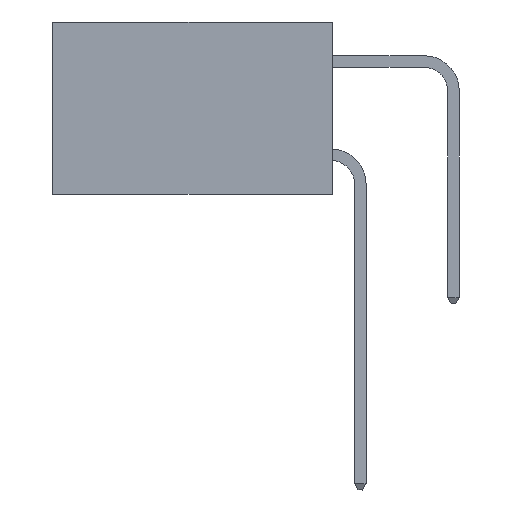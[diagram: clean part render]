
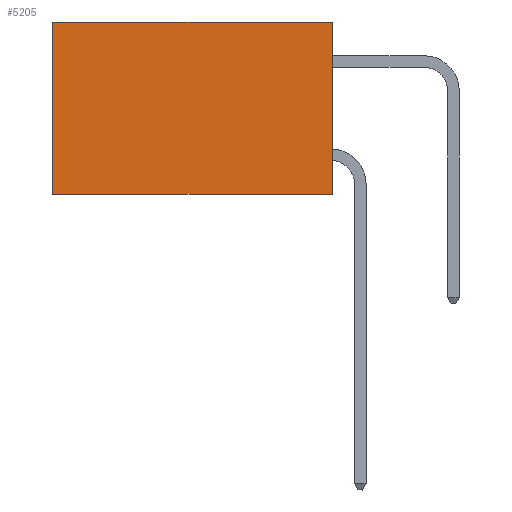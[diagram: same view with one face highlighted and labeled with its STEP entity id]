
A CAD part, left-side view. The second image highlights one B-rep face of the part: STEP entity #5205.
In plain terms, the highlighted planar face has unit normal (-1, 0, 0).
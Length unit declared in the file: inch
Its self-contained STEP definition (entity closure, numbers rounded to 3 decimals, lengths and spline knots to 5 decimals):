
#835 = LINE ( 'NONE', #24938, #24737 ) ;
#1611 = ORIENTED_EDGE ( 'NONE', *, *, #6503, .T. ) ;
#2766 = CARTESIAN_POINT ( 'NONE',  ( 0.298, 0., 0. ) ) ;
#2783 = LINE ( 'NONE', #4137, #17684 ) ;
#2809 = VERTEX_POINT ( 'NONE', #4584 ) ;
#3131 = VERTEX_POINT ( 'NONE', #24430 ) ;
#3649 = ORIENTED_EDGE ( 'NONE', *, *, #23106, .F. ) ;
#3903 = VECTOR ( 'NONE', #14174, 39.37008 ) ;
#4137 = CARTESIAN_POINT ( 'NONE',  ( 0.298, 0.6, 0. ) ) ;
#4584 = CARTESIAN_POINT ( 'NONE',  ( 0.298, 0.6, 0. ) ) ;
#4783 = EDGE_CURVE ( 'NONE', #2809, #14979, #2783, .T. ) ;
#5059 = ORIENTED_EDGE ( 'NONE', *, *, #8259, .F. ) ;
#5205 = ADVANCED_FACE ( 'NONE', ( #9171 ), #19211, .F. ) ;
#6503 = EDGE_CURVE ( 'NONE', #20878, #2809, #8493, .T. ) ;
#7600 = LINE ( 'NONE', #18352, #12145 ) ;
#8259 = EDGE_CURVE ( 'NONE', #3131, #14979, #835, .T. ) ;
#8493 = LINE ( 'NONE', #2766, #3903 ) ;
#9171 = FACE_OUTER_BOUND ( 'NONE', #19252, .T. ) ;
#11019 = CARTESIAN_POINT ( 'NONE',  ( 0.298, 0., 0. ) ) ;
#12145 = VECTOR ( 'NONE', #20284, 39.37008 ) ;
#12905 = ORIENTED_EDGE ( 'NONE', *, *, #4783, .T. ) ;
#14174 = DIRECTION ( 'NONE',  ( 0., 1., 0. ) ) ;
#14979 = VERTEX_POINT ( 'NONE', #20479 ) ;
#15081 = DIRECTION ( 'NONE',  ( 0., 1., 0. ) ) ;
#17684 = VECTOR ( 'NONE', #19784, 39.37008 ) ;
#18352 = CARTESIAN_POINT ( 'NONE',  ( 0.298, 0., 0. ) ) ;
#19097 = CARTESIAN_POINT ( 'NONE',  ( 0.298, 0., 0. ) ) ;
#19211 = PLANE ( 'NONE',  #24290 ) ;
#19252 = EDGE_LOOP ( 'NONE', ( #12905, #5059, #3649, #1611 ) ) ;
#19784 = DIRECTION ( 'NONE',  ( 0., 0., -1. ) ) ;
#20284 = DIRECTION ( 'NONE',  ( 0., 0., -1. ) ) ;
#20479 = CARTESIAN_POINT ( 'NONE',  ( 0.298, 0.6, -0.37 ) ) ;
#20878 = VERTEX_POINT ( 'NONE', #11019 ) ;
#21087 = DIRECTION ( 'NONE',  ( 0., 0., -1. ) ) ;
#22743 = DIRECTION ( 'NONE',  ( 1., 0., 0. ) ) ;
#23106 = EDGE_CURVE ( 'NONE', #20878, #3131, #7600, .T. ) ;
#24290 = AXIS2_PLACEMENT_3D ( 'NONE', #19097, #22743, #21087 ) ;
#24430 = CARTESIAN_POINT ( 'NONE',  ( 0.298, 0., -0.37 ) ) ;
#24737 = VECTOR ( 'NONE', #15081, 39.37008 ) ;
#24938 = CARTESIAN_POINT ( 'NONE',  ( 0.298, 0., -0.37 ) ) ;
